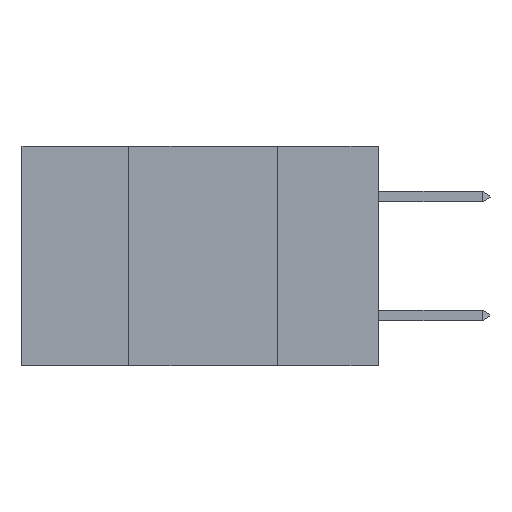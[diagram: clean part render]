
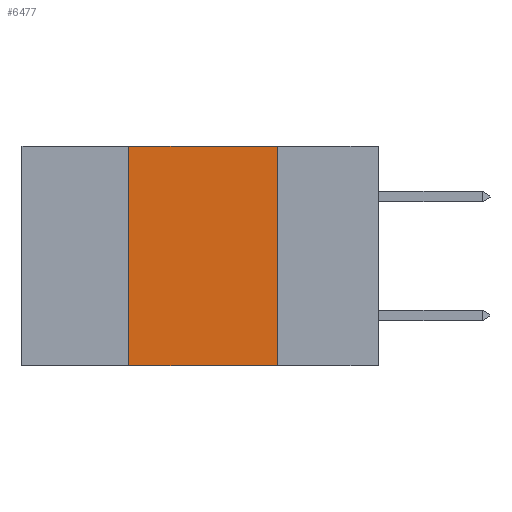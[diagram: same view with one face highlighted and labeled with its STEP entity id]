
A CAD part, left-side view. The second image highlights one B-rep face of the part: STEP entity #6477.
In plain terms, the highlighted planar face has unit normal (-1, 0, 0).
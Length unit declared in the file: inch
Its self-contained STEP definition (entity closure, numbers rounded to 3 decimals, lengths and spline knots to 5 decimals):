
#104 = CARTESIAN_POINT ( 'NONE',  ( 0., 0.42, 0. ) ) ;
#391 = CARTESIAN_POINT ( 'NONE',  ( 0., 0.17, 0. ) ) ;
#425 = EDGE_LOOP ( 'NONE', ( #17107, #16245, #6670, #6464 ) ) ;
#509 = EDGE_CURVE ( 'NONE', #10681, #10085, #11857, .T. ) ;
#923 = VECTOR ( 'NONE', #14568, 39.37008 ) ;
#1576 = VECTOR ( 'NONE', #8390, 39.37008 ) ;
#2400 = LINE ( 'NONE', #16888, #7850 ) ;
#2974 = VERTEX_POINT ( 'NONE', #6586 ) ;
#3622 = AXIS2_PLACEMENT_3D ( 'NONE', #15415, #13985, #12816 ) ;
#4068 = VERTEX_POINT ( 'NONE', #8947 ) ;
#5525 = CARTESIAN_POINT ( 'NONE',  ( 0., 0.17, 0. ) ) ;
#6050 = PLANE ( 'NONE',  #3622 ) ;
#6464 = ORIENTED_EDGE ( 'NONE', *, *, #12320, .T. ) ;
#6477 = ADVANCED_FACE ( 'NONE', ( #9662 ), #6050, .F. ) ;
#6586 = CARTESIAN_POINT ( 'NONE',  ( 0., 0.42, -0.37 ) ) ;
#6670 = ORIENTED_EDGE ( 'NONE', *, *, #15819, .F. ) ;
#7850 = VECTOR ( 'NONE', #11575, 39.37008 ) ;
#8257 = CARTESIAN_POINT ( 'NONE',  ( 0., 0.6, 0. ) ) ;
#8390 = DIRECTION ( 'NONE',  ( 0., 0., -1. ) ) ;
#8947 = CARTESIAN_POINT ( 'NONE',  ( 0., 0.17, -0.37 ) ) ;
#8954 = VECTOR ( 'NONE', #9495, 39.37008 ) ;
#9495 = DIRECTION ( 'NONE',  ( 0., -1., 0. ) ) ;
#9662 = FACE_OUTER_BOUND ( 'NONE', #425, .T. ) ;
#10085 = VERTEX_POINT ( 'NONE', #391 ) ;
#10681 = VERTEX_POINT ( 'NONE', #104 ) ;
#11164 = LINE ( 'NONE', #14397, #923 ) ;
#11575 = DIRECTION ( 'NONE',  ( 0., 0., 1. ) ) ;
#11857 = LINE ( 'NONE', #8257, #8954 ) ;
#12320 = EDGE_CURVE ( 'NONE', #2974, #4068, #11164, .T. ) ;
#12816 = DIRECTION ( 'NONE',  ( 0., 0., -1. ) ) ;
#13985 = DIRECTION ( 'NONE',  ( 1., 0., 0. ) ) ;
#14397 = CARTESIAN_POINT ( 'NONE',  ( 0., 0.6, -0.37 ) ) ;
#14568 = DIRECTION ( 'NONE',  ( 0., -1., 0. ) ) ;
#14968 = LINE ( 'NONE', #5525, #1576 ) ;
#15415 = CARTESIAN_POINT ( 'NONE',  ( 0., 0.6, 0. ) ) ;
#15564 = EDGE_CURVE ( 'NONE', #10085, #4068, #14968, .T. ) ;
#15819 = EDGE_CURVE ( 'NONE', #2974, #10681, #2400, .T. ) ;
#16245 = ORIENTED_EDGE ( 'NONE', *, *, #509, .F. ) ;
#16888 = CARTESIAN_POINT ( 'NONE',  ( 0., 0.42, 0. ) ) ;
#17107 = ORIENTED_EDGE ( 'NONE', *, *, #15564, .F. ) ;
